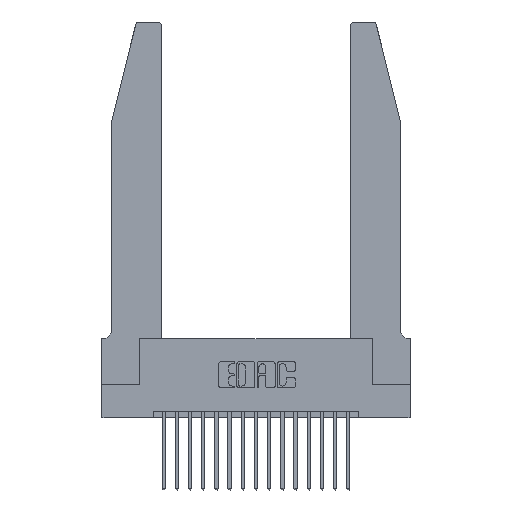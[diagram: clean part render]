
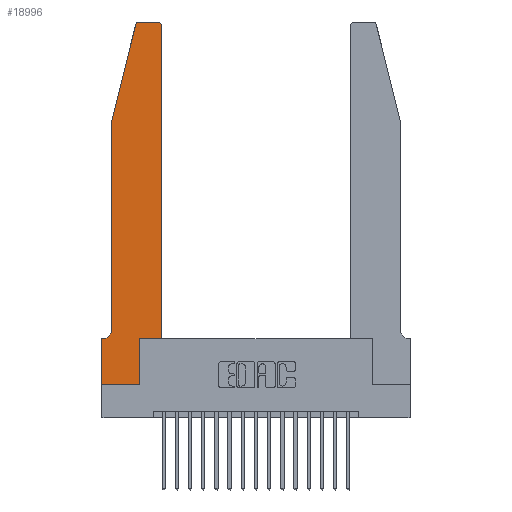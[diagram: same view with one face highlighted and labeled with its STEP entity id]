
A CAD part, top view. The second image highlights one B-rep face of the part: STEP entity #18996.
In plain terms, the highlighted planar face has unit normal (0, 0, 1).
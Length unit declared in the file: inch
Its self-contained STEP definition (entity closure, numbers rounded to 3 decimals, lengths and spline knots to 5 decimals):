
#14 = DIRECTION ( 'NONE',  ( 0., -1., 0. ) ) ;
#283 = LINE ( 'NONE', #3445, #16513 ) ;
#330 = DIRECTION ( 'NONE',  ( 0., 1., 0. ) ) ;
#422 = EDGE_CURVE ( 'NONE', #14263, #3059, #11431, .T. ) ;
#637 = DIRECTION ( 'NONE',  ( 1., 0., 0. ) ) ;
#829 = VERTEX_POINT ( 'NONE', #19466 ) ;
#1014 = LINE ( 'NONE', #9827, #20158 ) ;
#1129 = DIRECTION ( 'NONE',  ( -1., 0., 0. ) ) ;
#1234 = ORIENTED_EDGE ( 'NONE', *, *, #5330, .T. ) ;
#1351 = ORIENTED_EDGE ( 'NONE', *, *, #16073, .T. ) ;
#1538 = VERTEX_POINT ( 'NONE', #11342 ) ;
#1886 = VECTOR ( 'NONE', #8664, 39.37008 ) ;
#1935 = DIRECTION ( 'NONE',  ( 1., 0., 0. ) ) ;
#2080 = LINE ( 'NONE', #6794, #6319 ) ;
#3020 = CARTESIAN_POINT ( 'NONE',  ( 0., 0.35, 0.37 ) ) ;
#3059 = VERTEX_POINT ( 'NONE', #14563 ) ;
#3374 = LINE ( 'NONE', #5980, #11248 ) ;
#3445 = CARTESIAN_POINT ( 'NONE',  ( 0., 0., 0.37 ) ) ;
#3804 = DIRECTION ( 'NONE',  ( 0., -1., 0. ) ) ;
#3875 = CARTESIAN_POINT ( 'NONE',  ( 0.4205, 2.72, 0.37 ) ) ;
#3920 = CARTESIAN_POINT ( 'NONE',  ( 0.2865, 0.35, 0.37 ) ) ;
#4018 = VERTEX_POINT ( 'NONE', #3920 ) ;
#4043 = CARTESIAN_POINT ( 'NONE',  ( 0.284, 2.72, 0.37 ) ) ;
#4386 = DIRECTION ( 'NONE',  ( 0., 1., 0. ) ) ;
#4663 = AXIS2_PLACEMENT_3D ( 'NONE', #4043, #14954, #5660 ) ;
#5330 = EDGE_CURVE ( 'NONE', #19886, #14280, #283, .T. ) ;
#5412 = CARTESIAN_POINT ( 'NONE',  ( 0., 0., 0.37 ) ) ;
#5536 = CARTESIAN_POINT ( 'NONE',  ( 0.0755, 0.42, 0.37 ) ) ;
#5648 = DIRECTION ( 'NONE',  ( 0., 0., 1. ) ) ;
#5660 = DIRECTION ( 'NONE',  ( 1., 0., 0. ) ) ;
#5980 = CARTESIAN_POINT ( 'NONE',  ( 0.0755, 0.35, 0.37 ) ) ;
#6319 = VECTOR ( 'NONE', #330, 39.37008 ) ;
#6335 = CIRCLE ( 'NONE', #4663, 0.03 ) ;
#6495 = CARTESIAN_POINT ( 'NONE',  ( 0.2865, 0., 0.37 ) ) ;
#6777 = EDGE_CURVE ( 'NONE', #19219, #19886, #10844, .T. ) ;
#6786 = CARTESIAN_POINT ( 'NONE',  ( 0.2605, 2.75, 0.37 ) ) ;
#6794 = CARTESIAN_POINT ( 'NONE',  ( 0.4505, 0.35, 0.37 ) ) ;
#6859 = DIRECTION ( 'NONE',  ( -1., 0., 0. ) ) ;
#6884 = EDGE_LOOP ( 'NONE', ( #10396, #10379, #9168, #7349, #1351, #9477, #16703, #1234, #7511, #19820, #12537, #19594 ) ) ;
#7159 = VECTOR ( 'NONE', #4386, 39.37008 ) ;
#7296 = VERTEX_POINT ( 'NONE', #5536 ) ;
#7349 = ORIENTED_EDGE ( 'NONE', *, *, #11964, .T. ) ;
#7466 = VECTOR ( 'NONE', #14, 39.37008 ) ;
#7511 = ORIENTED_EDGE ( 'NONE', *, *, #19216, .T. ) ;
#7944 = DIRECTION ( 'NONE',  ( 0., 0., -1. ) ) ;
#8122 = CARTESIAN_POINT ( 'NONE',  ( 0.0055, 0.35, 0.37 ) ) ;
#8600 = EDGE_CURVE ( 'NONE', #14976, #19219, #3374, .T. ) ;
#8664 = DIRECTION ( 'NONE',  ( -0.239, -0.971, 0. ) ) ;
#9168 = ORIENTED_EDGE ( 'NONE', *, *, #13434, .T. ) ;
#9233 = AXIS2_PLACEMENT_3D ( 'NONE', #3875, #5648, #17514 ) ;
#9410 = EDGE_CURVE ( 'NONE', #13559, #10225, #6335, .T. ) ;
#9477 = ORIENTED_EDGE ( 'NONE', *, *, #8600, .T. ) ;
#9666 = CARTESIAN_POINT ( 'NONE',  ( 0.0755, 2., 0.37 ) ) ;
#9827 = CARTESIAN_POINT ( 'NONE',  ( 0.4505, 0.35, 0.37 ) ) ;
#10222 = DIRECTION ( 'NONE',  ( 0., 0., 1. ) ) ;
#10225 = VERTEX_POINT ( 'NONE', #13247 ) ;
#10366 = VECTOR ( 'NONE', #3804, 39.37008 ) ;
#10379 = ORIENTED_EDGE ( 'NONE', *, *, #9410, .T. ) ;
#10396 = ORIENTED_EDGE ( 'NONE', *, *, #12119, .T. ) ;
#10581 = FACE_OUTER_BOUND ( 'NONE', #6884, .T. ) ;
#10844 = LINE ( 'NONE', #5412, #10366 ) ;
#11248 = VECTOR ( 'NONE', #1129, 39.37008 ) ;
#11342 = CARTESIAN_POINT ( 'NONE',  ( 0.4505, 0.35, 0.37 ) ) ;
#11431 = CIRCLE ( 'NONE', #9233, 0.03 ) ;
#11964 = EDGE_CURVE ( 'NONE', #829, #7296, #15653, .T. ) ;
#12119 = EDGE_CURVE ( 'NONE', #3059, #13559, #16337, .T. ) ;
#12311 = VECTOR ( 'NONE', #6859, 39.37008 ) ;
#12426 = CARTESIAN_POINT ( 'NONE',  ( 0.2865, 0.35, 0.37 ) ) ;
#12537 = ORIENTED_EDGE ( 'NONE', *, *, #15657, .T. ) ;
#12600 = CARTESIAN_POINT ( 'NONE',  ( 0., 0., 0.37 ) ) ;
#13247 = CARTESIAN_POINT ( 'NONE',  ( 0.25487, 2.72718, 0.37 ) ) ;
#13260 = CARTESIAN_POINT ( 'NONE',  ( 0.0755, 2., 0.37 ) ) ;
#13434 = EDGE_CURVE ( 'NONE', #10225, #829, #13440, .T. ) ;
#13440 = LINE ( 'NONE', #13260, #1886 ) ;
#13559 = VERTEX_POINT ( 'NONE', #16541 ) ;
#14226 = CARTESIAN_POINT ( 'NONE',  ( 0.4505, 2.72, 0.37 ) ) ;
#14263 = VERTEX_POINT ( 'NONE', #14226 ) ;
#14280 = VERTEX_POINT ( 'NONE', #6495 ) ;
#14386 = AXIS2_PLACEMENT_3D ( 'NONE', #17124, #7944, #18642 ) ;
#14563 = CARTESIAN_POINT ( 'NONE',  ( 0.4205, 2.75, 0.37 ) ) ;
#14774 = CARTESIAN_POINT ( 'NONE',  ( 0., 0.35, 0.37 ) ) ;
#14954 = DIRECTION ( 'NONE',  ( 0., 0., 1. ) ) ;
#14976 = VERTEX_POINT ( 'NONE', #8122 ) ;
#15042 = EDGE_CURVE ( 'NONE', #4018, #1538, #1014, .T. ) ;
#15653 = LINE ( 'NONE', #9666, #7466 ) ;
#15657 = EDGE_CURVE ( 'NONE', #1538, #14263, #2080, .T. ) ;
#16073 = EDGE_CURVE ( 'NONE', #7296, #14976, #18997, .T. ) ;
#16337 = LINE ( 'NONE', #6786, #12311 ) ;
#16513 = VECTOR ( 'NONE', #17396, 39.37008 ) ;
#16541 = CARTESIAN_POINT ( 'NONE',  ( 0.284, 2.75, 0.37 ) ) ;
#16703 = ORIENTED_EDGE ( 'NONE', *, *, #6777, .T. ) ;
#17124 = CARTESIAN_POINT ( 'NONE',  ( 0.0055, 0.42, 0.37 ) ) ;
#17396 = DIRECTION ( 'NONE',  ( 1., 0., 0. ) ) ;
#17514 = DIRECTION ( 'NONE',  ( 1., 0., 0. ) ) ;
#18642 = DIRECTION ( 'NONE',  ( -1., 0., 0. ) ) ;
#18872 = LINE ( 'NONE', #12426, #7159 ) ;
#18996 = ADVANCED_FACE ( 'NONE', ( #10581 ), #19298, .T. ) ;
#18997 = CIRCLE ( 'NONE', #14386, 0.07 ) ;
#19216 = EDGE_CURVE ( 'NONE', #14280, #4018, #18872, .T. ) ;
#19219 = VERTEX_POINT ( 'NONE', #3020 ) ;
#19298 = PLANE ( 'NONE',  #20051 ) ;
#19466 = CARTESIAN_POINT ( 'NONE',  ( 0.0755, 2., 0.37 ) ) ;
#19594 = ORIENTED_EDGE ( 'NONE', *, *, #422, .T. ) ;
#19820 = ORIENTED_EDGE ( 'NONE', *, *, #15042, .T. ) ;
#19886 = VERTEX_POINT ( 'NONE', #12600 ) ;
#20051 = AXIS2_PLACEMENT_3D ( 'NONE', #14774, #10222, #637 ) ;
#20158 = VECTOR ( 'NONE', #1935, 39.37008 ) ;
